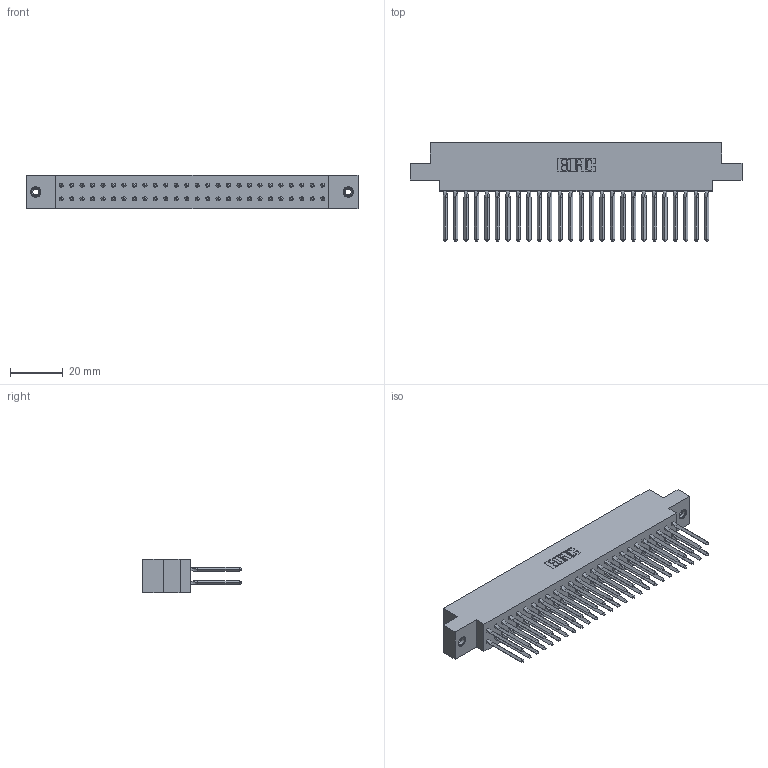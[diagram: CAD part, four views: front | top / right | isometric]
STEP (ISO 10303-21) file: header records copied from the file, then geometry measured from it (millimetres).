
FILE_DESCRIPTION (( 'STEP AP203' ), '1' );
FILE_NAME ('317-052-542-878.STEP', '2020-02-28T03:37:45', ( '' ), ( '' ), 'SwSTEP 2.0', 'SolidWorks 2016', '' );
FILE_SCHEMA (( 'CONFIG_CONTROL_DESIGN' ));
Length unit declared in the file: inch
Products named in the file (4): 317-290-003_542; 317-052-542-878; 317 Part_.156 Dia - TI; 345-250-001_345-250-003-102
Assembly tree (55 placements, depth 2):
  317-052-542-878
    317 Part_.156 Dia - TI
    317-290-003_542  x52
    345-250-001_345-250-003-102  x2
Bounding box: 125.73 x 37.34 x 12.7 mm (x, y, z)
Volume: 20075.7 mm3; surface area: 27426.2 mm2
Topology: 55 solids, 55 shells, 3126 faces, 8731 edges, 5570 vertices
Faces by surface type: plane 2482, cylinder 420, bspline 208, cone 12, torus 4
Entity records: 40018 total; most frequent: CARTESIAN_POINT 7200, ORIENTED_EDGE 6856, DIRECTION 5834, EDGE_CURVE 3428, LINE 3238, VECTOR 3238, VERTEX_POINT 2276, AXIS2_PLACEMENT_3D 1298
